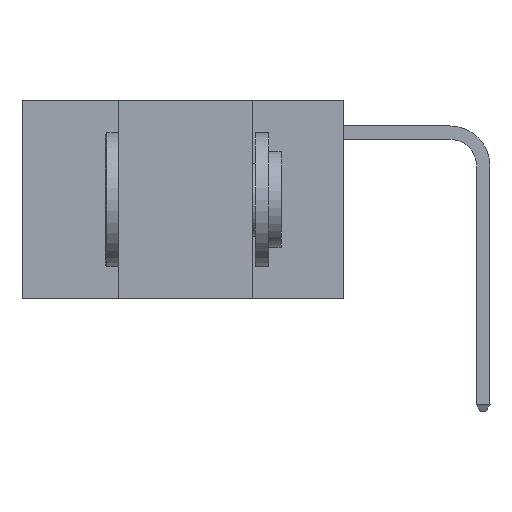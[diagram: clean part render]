
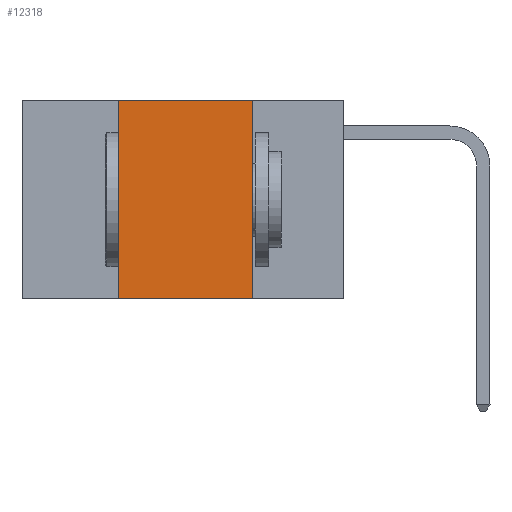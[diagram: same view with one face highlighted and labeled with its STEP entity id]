
A CAD part, left-side view. The second image highlights one B-rep face of the part: STEP entity #12318.
In plain terms, the highlighted planar face has unit normal (-1, 0, 0).
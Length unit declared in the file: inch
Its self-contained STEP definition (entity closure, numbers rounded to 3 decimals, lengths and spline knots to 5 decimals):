
#110 = VERTEX_POINT ( 'NONE', #12542 ) ;
#522 = CARTESIAN_POINT ( 'NONE',  ( 0., 0.6, 0. ) ) ;
#877 = VECTOR ( 'NONE', #4643, 39.37008 ) ;
#1522 = AXIS2_PLACEMENT_3D ( 'NONE', #522, #11291, #12529 ) ;
#2514 = EDGE_CURVE ( 'NONE', #110, #10442, #8816, .T. ) ;
#2658 = CARTESIAN_POINT ( 'NONE',  ( 0., 0.17, 0. ) ) ;
#2958 = LINE ( 'NONE', #5812, #13581 ) ;
#3237 = EDGE_LOOP ( 'NONE', ( #15369, #6413, #12818, #7382 ) ) ;
#4643 = DIRECTION ( 'NONE',  ( 0., 0., 1. ) ) ;
#4764 = PLANE ( 'NONE',  #1522 ) ;
#4855 = VECTOR ( 'NONE', #16624, 39.37008 ) ;
#5812 = CARTESIAN_POINT ( 'NONE',  ( 0., 0.17, 0. ) ) ;
#6413 = ORIENTED_EDGE ( 'NONE', *, *, #2514, .F. ) ;
#6576 = EDGE_CURVE ( 'NONE', #16498, #110, #14034, .T. ) ;
#7237 = DIRECTION ( 'NONE',  ( 0., 0., -1. ) ) ;
#7382 = ORIENTED_EDGE ( 'NONE', *, *, #17619, .T. ) ;
#8522 = VERTEX_POINT ( 'NONE', #10530 ) ;
#8816 = LINE ( 'NONE', #11142, #4855 ) ;
#10442 = VERTEX_POINT ( 'NONE', #2658 ) ;
#10530 = CARTESIAN_POINT ( 'NONE',  ( 0., 0.17, -0.37 ) ) ;
#10532 = LINE ( 'NONE', #14649, #16199 ) ;
#11142 = CARTESIAN_POINT ( 'NONE',  ( 0., 0.6, 0. ) ) ;
#11291 = DIRECTION ( 'NONE',  ( 1., 0., 0. ) ) ;
#12318 = ADVANCED_FACE ( 'NONE', ( #17057 ), #4764, .F. ) ;
#12529 = DIRECTION ( 'NONE',  ( 0., 0., -1. ) ) ;
#12542 = CARTESIAN_POINT ( 'NONE',  ( 0., 0.42, 0. ) ) ;
#12818 = ORIENTED_EDGE ( 'NONE', *, *, #6576, .F. ) ;
#13187 = CARTESIAN_POINT ( 'NONE',  ( 0., 0.42, -0.37 ) ) ;
#13581 = VECTOR ( 'NONE', #7237, 39.37008 ) ;
#14034 = LINE ( 'NONE', #14127, #877 ) ;
#14127 = CARTESIAN_POINT ( 'NONE',  ( 0., 0.42, 0. ) ) ;
#14649 = CARTESIAN_POINT ( 'NONE',  ( 0., 0.6, -0.37 ) ) ;
#15369 = ORIENTED_EDGE ( 'NONE', *, *, #17029, .F. ) ;
#16199 = VECTOR ( 'NONE', #16273, 39.37008 ) ;
#16273 = DIRECTION ( 'NONE',  ( 0., -1., 0. ) ) ;
#16498 = VERTEX_POINT ( 'NONE', #13187 ) ;
#16624 = DIRECTION ( 'NONE',  ( 0., -1., 0. ) ) ;
#17029 = EDGE_CURVE ( 'NONE', #10442, #8522, #2958, .T. ) ;
#17057 = FACE_OUTER_BOUND ( 'NONE', #3237, .T. ) ;
#17619 = EDGE_CURVE ( 'NONE', #16498, #8522, #10532, .T. ) ;
